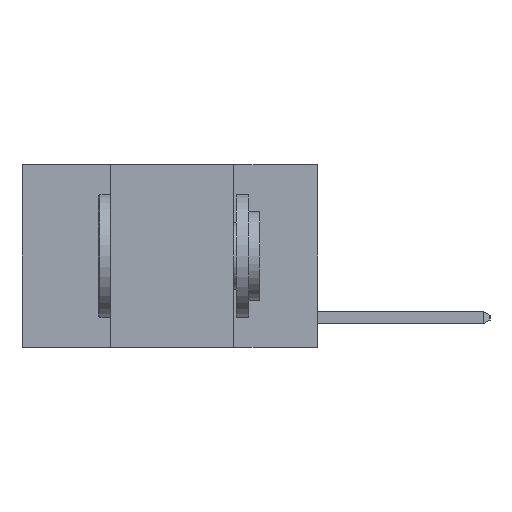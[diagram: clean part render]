
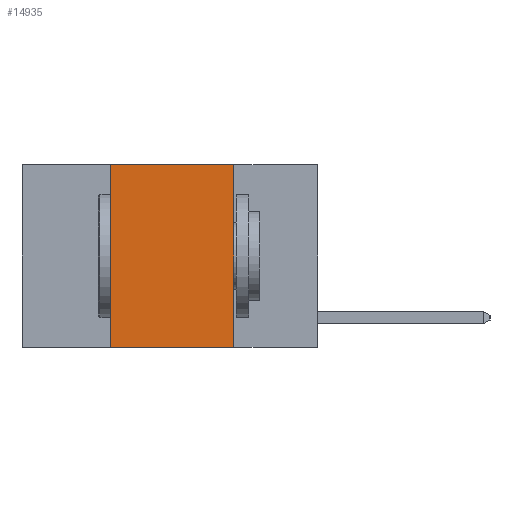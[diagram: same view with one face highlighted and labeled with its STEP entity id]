
A CAD part, left-side view. The second image highlights one B-rep face of the part: STEP entity #14935.
In plain terms, the highlighted planar face has unit normal (-1, 0, 0).
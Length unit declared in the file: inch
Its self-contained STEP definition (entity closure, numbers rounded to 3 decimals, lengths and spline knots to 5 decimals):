
#58 = CARTESIAN_POINT ( 'NONE',  ( 0., 0.6, 0. ) ) ;
#444 = VERTEX_POINT ( 'NONE', #15237 ) ;
#475 = AXIS2_PLACEMENT_3D ( 'NONE', #58, #9638, #1508 ) ;
#711 = VECTOR ( 'NONE', #15468, 39.37008 ) ;
#1508 = DIRECTION ( 'NONE',  ( 0., 0., -1. ) ) ;
#2387 = DIRECTION ( 'NONE',  ( 0., -1., 0. ) ) ;
#2434 = ORIENTED_EDGE ( 'NONE', *, *, #5604, .F. ) ;
#2927 = DIRECTION ( 'NONE',  ( 0., 0., 1. ) ) ;
#2983 = CARTESIAN_POINT ( 'NONE',  ( 0., 0.42, 0. ) ) ;
#3363 = EDGE_LOOP ( 'NONE', ( #2434, #3659, #9507, #9713 ) ) ;
#3642 = LINE ( 'NONE', #13003, #7292 ) ;
#3659 = ORIENTED_EDGE ( 'NONE', *, *, #8485, .F. ) ;
#5604 = EDGE_CURVE ( 'NONE', #444, #15401, #16663, .T. ) ;
#6227 = LINE ( 'NONE', #2983, #9296 ) ;
#6467 = CARTESIAN_POINT ( 'NONE',  ( 0., 0.17, 0. ) ) ;
#7292 = VECTOR ( 'NONE', #2387, 39.37008 ) ;
#8485 = EDGE_CURVE ( 'NONE', #8763, #444, #3642, .T. ) ;
#8763 = VERTEX_POINT ( 'NONE', #12210 ) ;
#9296 = VECTOR ( 'NONE', #2927, 39.37008 ) ;
#9507 = ORIENTED_EDGE ( 'NONE', *, *, #16477, .F. ) ;
#9638 = DIRECTION ( 'NONE',  ( 1., 0., 0. ) ) ;
#9713 = ORIENTED_EDGE ( 'NONE', *, *, #15339, .T. ) ;
#10204 = FACE_OUTER_BOUND ( 'NONE', #3363, .T. ) ;
#10344 = DIRECTION ( 'NONE',  ( 0., -1., 0. ) ) ;
#10524 = VERTEX_POINT ( 'NONE', #15890 ) ;
#10993 = LINE ( 'NONE', #15392, #14372 ) ;
#12210 = CARTESIAN_POINT ( 'NONE',  ( 0., 0.42, 0. ) ) ;
#13003 = CARTESIAN_POINT ( 'NONE',  ( 0., 0.6, 0. ) ) ;
#14287 = CARTESIAN_POINT ( 'NONE',  ( 0., 0.17, -0.37 ) ) ;
#14372 = VECTOR ( 'NONE', #10344, 39.37008 ) ;
#14753 = PLANE ( 'NONE',  #475 ) ;
#14935 = ADVANCED_FACE ( 'NONE', ( #10204 ), #14753, .F. ) ;
#15237 = CARTESIAN_POINT ( 'NONE',  ( 0., 0.17, 0. ) ) ;
#15339 = EDGE_CURVE ( 'NONE', #10524, #15401, #10993, .T. ) ;
#15392 = CARTESIAN_POINT ( 'NONE',  ( 0., 0.6, -0.37 ) ) ;
#15401 = VERTEX_POINT ( 'NONE', #14287 ) ;
#15468 = DIRECTION ( 'NONE',  ( 0., 0., -1. ) ) ;
#15890 = CARTESIAN_POINT ( 'NONE',  ( 0., 0.42, -0.37 ) ) ;
#16477 = EDGE_CURVE ( 'NONE', #10524, #8763, #6227, .T. ) ;
#16663 = LINE ( 'NONE', #6467, #711 ) ;
